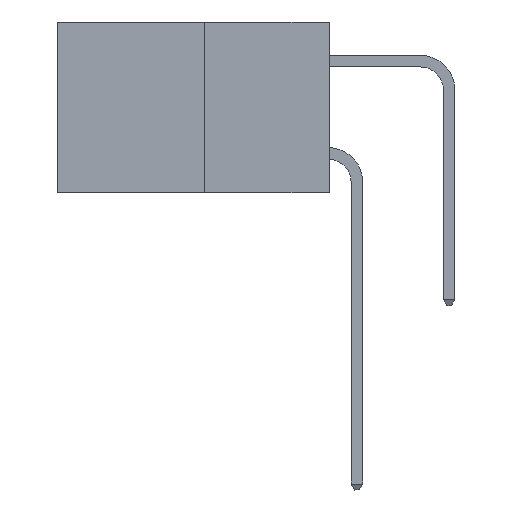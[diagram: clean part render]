
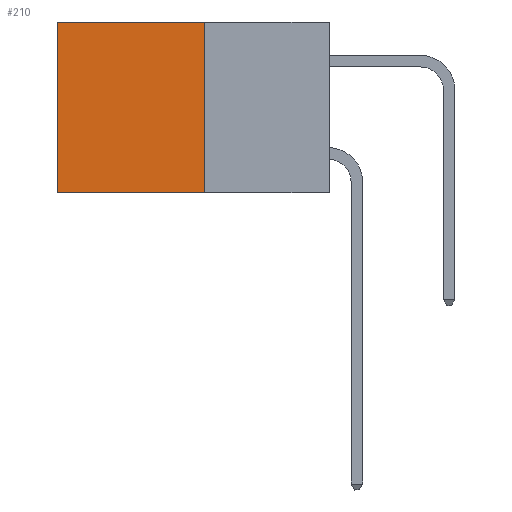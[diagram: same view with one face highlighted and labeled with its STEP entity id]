
A CAD part, left-side view. The second image highlights one B-rep face of the part: STEP entity #210.
In plain terms, the highlighted planar face has unit normal (-1, 0, 0).
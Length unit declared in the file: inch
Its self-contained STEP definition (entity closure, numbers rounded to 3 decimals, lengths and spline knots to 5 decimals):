
#132 = CARTESIAN_POINT ( 'NONE',  ( 0.277, 0.27, 0. ) ) ;
#210 = ADVANCED_FACE ( 'NONE', ( #10098 ), #3712, .F. ) ;
#272 = EDGE_CURVE ( 'NONE', #1473, #2358, #11221, .T. ) ;
#420 = VECTOR ( 'NONE', #2097, 39.37008 ) ;
#1143 = CARTESIAN_POINT ( 'NONE',  ( 0.277, 0.27, -0.37 ) ) ;
#1450 = DIRECTION ( 'NONE',  ( 0., 0., -1. ) ) ;
#1473 = VERTEX_POINT ( 'NONE', #8528 ) ;
#2097 = DIRECTION ( 'NONE',  ( 0., 0., -1. ) ) ;
#2103 = DIRECTION ( 'NONE',  ( 0., 1., 0. ) ) ;
#2358 = VERTEX_POINT ( 'NONE', #7986 ) ;
#2577 = DIRECTION ( 'NONE',  ( 1., 0., 0. ) ) ;
#2910 = CARTESIAN_POINT ( 'NONE',  ( 0.277, 0.27, -0.37 ) ) ;
#3712 = PLANE ( 'NONE',  #6250 ) ;
#4067 = VECTOR ( 'NONE', #2103, 39.37008 ) ;
#4720 = VECTOR ( 'NONE', #6828, 39.37008 ) ;
#6250 = AXIS2_PLACEMENT_3D ( 'NONE', #9239, #2577, #1450 ) ;
#6376 = EDGE_CURVE ( 'NONE', #2358, #9131, #9248, .T. ) ;
#6742 = ORIENTED_EDGE ( 'NONE', *, *, #6376, .T. ) ;
#6828 = DIRECTION ( 'NONE',  ( 0., 0., -1. ) ) ;
#7026 = ORIENTED_EDGE ( 'NONE', *, *, #7242, .F. ) ;
#7242 = EDGE_CURVE ( 'NONE', #1473, #10014, #9489, .T. ) ;
#7676 = VECTOR ( 'NONE', #9606, 39.37008 ) ;
#7986 = CARTESIAN_POINT ( 'NONE',  ( 0.277, 0.59, 0. ) ) ;
#8338 = CARTESIAN_POINT ( 'NONE',  ( 0.277, 0.59, -0.37 ) ) ;
#8528 = CARTESIAN_POINT ( 'NONE',  ( 0.277, 0.27, 0. ) ) ;
#8853 = ORIENTED_EDGE ( 'NONE', *, *, #272, .T. ) ;
#9049 = CARTESIAN_POINT ( 'NONE',  ( 0.277, 0.27, -0.37 ) ) ;
#9131 = VERTEX_POINT ( 'NONE', #10010 ) ;
#9239 = CARTESIAN_POINT ( 'NONE',  ( 0.277, 0.27, -0.37 ) ) ;
#9248 = LINE ( 'NONE', #8338, #4720 ) ;
#9482 = ORIENTED_EDGE ( 'NONE', *, *, #10050, .F. ) ;
#9489 = LINE ( 'NONE', #9049, #420 ) ;
#9606 = DIRECTION ( 'NONE',  ( 0., 1., 0. ) ) ;
#9999 = EDGE_LOOP ( 'NONE', ( #6742, #9482, #7026, #8853 ) ) ;
#10010 = CARTESIAN_POINT ( 'NONE',  ( 0.277, 0.59, -0.37 ) ) ;
#10014 = VERTEX_POINT ( 'NONE', #2910 ) ;
#10050 = EDGE_CURVE ( 'NONE', #10014, #9131, #11072, .T. ) ;
#10098 = FACE_OUTER_BOUND ( 'NONE', #9999, .T. ) ;
#11072 = LINE ( 'NONE', #1143, #4067 ) ;
#11221 = LINE ( 'NONE', #132, #7676 ) ;
